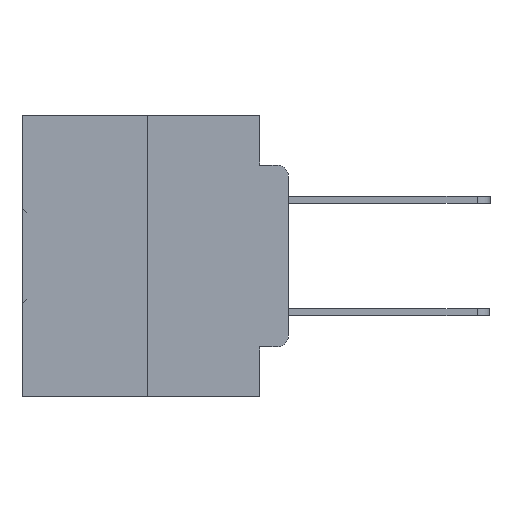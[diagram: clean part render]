
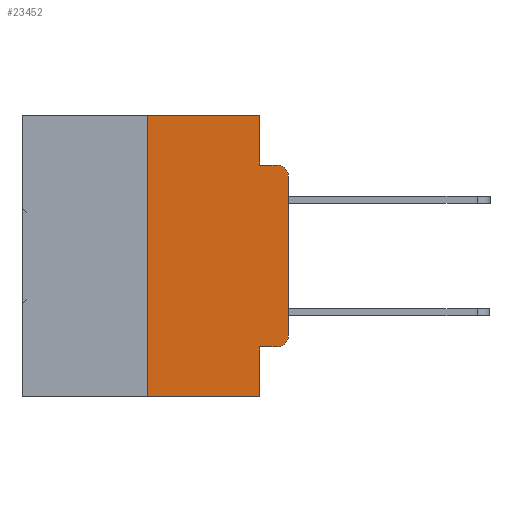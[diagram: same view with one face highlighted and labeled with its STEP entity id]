
A CAD part, left-side view. The second image highlights one B-rep face of the part: STEP entity #23452.
In plain terms, the highlighted planar face has unit normal (-1, 0, 0).
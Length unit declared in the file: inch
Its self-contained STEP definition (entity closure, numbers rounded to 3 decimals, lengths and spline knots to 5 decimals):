
#125 = DIRECTION ( 'NONE',  ( 0., 0., -1. ) ) ;
#289 = VERTEX_POINT ( 'NONE', #16838 ) ;
#683 = LINE ( 'NONE', #22170, #1549 ) ;
#1359 = VERTEX_POINT ( 'NONE', #10719 ) ;
#1549 = VECTOR ( 'NONE', #3094, 39.37008 ) ;
#2025 = EDGE_CURVE ( 'NONE', #9651, #2860, #10734, .T. ) ;
#2363 = DIRECTION ( 'NONE',  ( 0., 0., 1. ) ) ;
#2707 = DIRECTION ( 'NONE',  ( 0., 0., -1. ) ) ;
#2860 = VERTEX_POINT ( 'NONE', #33324 ) ;
#3094 = DIRECTION ( 'NONE',  ( 0., -1., 0. ) ) ;
#3536 = EDGE_CURVE ( 'NONE', #31748, #29244, #20817, .T. ) ;
#4374 = AXIS2_PLACEMENT_3D ( 'NONE', #27597, #30300, #14190 ) ;
#4842 = ORIENTED_EDGE ( 'NONE', *, *, #16041, .T. ) ;
#4948 = CARTESIAN_POINT ( 'NONE',  ( 0., 0.02, -0.1085 ) ) ;
#5234 = LINE ( 'NONE', #31749, #26900 ) ;
#5281 = ORIENTED_EDGE ( 'NONE', *, *, #9708, .F. ) ;
#5683 = EDGE_LOOP ( 'NONE', ( #11292, #4842, #21050, #22722, #11728, #5281, #7027, #21469, #13063, #28225 ) ) ;
#5907 = PLANE ( 'NONE',  #4374 ) ;
#6290 = EDGE_CURVE ( 'NONE', #289, #31748, #683, .T. ) ;
#6337 = VECTOR ( 'NONE', #11534, 39.37008 ) ;
#6367 = VERTEX_POINT ( 'NONE', #27935 ) ;
#6735 = CARTESIAN_POINT ( 'NONE',  ( 0., 0.473, -0.5 ) ) ;
#7027 = ORIENTED_EDGE ( 'NONE', *, *, #26591, .T. ) ;
#7116 = VECTOR ( 'NONE', #9480, 39.37008 ) ;
#7209 = AXIS2_PLACEMENT_3D ( 'NONE', #30746, #14648, #33377 ) ;
#7302 = EDGE_CURVE ( 'NONE', #6367, #24954, #22806, .T. ) ;
#8119 = LINE ( 'NONE', #30561, #21718 ) ;
#8547 = VERTEX_POINT ( 'NONE', #34655 ) ;
#9480 = DIRECTION ( 'NONE',  ( 0., -1., 0. ) ) ;
#9651 = VERTEX_POINT ( 'NONE', #34145 ) ;
#9708 = EDGE_CURVE ( 'NONE', #8547, #289, #5234, .T. ) ;
#9739 = CARTESIAN_POINT ( 'NONE',  ( 0., 0.051, 0. ) ) ;
#9971 = AXIS2_PLACEMENT_3D ( 'NONE', #4948, #16576, #125 ) ;
#10719 = CARTESIAN_POINT ( 'NONE',  ( 0., 0.02, -0.4115 ) ) ;
#10734 = LINE ( 'NONE', #18844, #25955 ) ;
#11292 = ORIENTED_EDGE ( 'NONE', *, *, #2025, .T. ) ;
#11534 = DIRECTION ( 'NONE',  ( 0., 0., -1. ) ) ;
#11652 = EDGE_CURVE ( 'NONE', #1359, #9651, #31369, .T. ) ;
#11728 = ORIENTED_EDGE ( 'NONE', *, *, #6290, .F. ) ;
#12935 = DIRECTION ( 'NONE',  ( 0., 0., 1. ) ) ;
#13063 = ORIENTED_EDGE ( 'NONE', *, *, #29251, .T. ) ;
#14190 = DIRECTION ( 'NONE',  ( 0., 0., -1. ) ) ;
#14440 = CARTESIAN_POINT ( 'NONE',  ( 0., 0.051, 0. ) ) ;
#14648 = DIRECTION ( 'NONE',  ( -1., 0., 0. ) ) ;
#15057 = LINE ( 'NONE', #19139, #29360 ) ;
#16041 = EDGE_CURVE ( 'NONE', #2860, #29183, #16885, .T. ) ;
#16576 = DIRECTION ( 'NONE',  ( -1., 0., 0. ) ) ;
#16838 = CARTESIAN_POINT ( 'NONE',  ( 0., 0.25, 0. ) ) ;
#16885 = CIRCLE ( 'NONE', #9971, 0.02 ) ;
#18844 = CARTESIAN_POINT ( 'NONE',  ( 0., 0., 0. ) ) ;
#18910 = CARTESIAN_POINT ( 'NONE',  ( 0., 0.02, -0.0885 ) ) ;
#19139 = CARTESIAN_POINT ( 'NONE',  ( 0., 0.051, -0.4115 ) ) ;
#20817 = LINE ( 'NONE', #14440, #6337 ) ;
#21050 = ORIENTED_EDGE ( 'NONE', *, *, #21754, .F. ) ;
#21469 = ORIENTED_EDGE ( 'NONE', *, *, #7302, .F. ) ;
#21718 = VECTOR ( 'NONE', #33205, 39.37008 ) ;
#21754 = EDGE_CURVE ( 'NONE', #29244, #29183, #8119, .T. ) ;
#21961 = VECTOR ( 'NONE', #2707, 39.37008 ) ;
#22170 = CARTESIAN_POINT ( 'NONE',  ( 0., 0.473, 0. ) ) ;
#22722 = ORIENTED_EDGE ( 'NONE', *, *, #3536, .F. ) ;
#22806 = LINE ( 'NONE', #32442, #21961 ) ;
#23452 = ADVANCED_FACE ( 'NONE', ( #26668 ), #5907, .F. ) ;
#24312 = DIRECTION ( 'NONE',  ( 0., -1., 0. ) ) ;
#24434 = CARTESIAN_POINT ( 'NONE',  ( 0., 0.051, -0.0885 ) ) ;
#24954 = VERTEX_POINT ( 'NONE', #31985 ) ;
#25955 = VECTOR ( 'NONE', #2363, 39.37008 ) ;
#26591 = EDGE_CURVE ( 'NONE', #8547, #24954, #28718, .T. ) ;
#26668 = FACE_OUTER_BOUND ( 'NONE', #5683, .T. ) ;
#26900 = VECTOR ( 'NONE', #12935, 39.37008 ) ;
#27597 = CARTESIAN_POINT ( 'NONE',  ( 0., 0.473, 0. ) ) ;
#27935 = CARTESIAN_POINT ( 'NONE',  ( 0., 0.051, -0.4115 ) ) ;
#28225 = ORIENTED_EDGE ( 'NONE', *, *, #11652, .T. ) ;
#28718 = LINE ( 'NONE', #6735, #7116 ) ;
#29183 = VERTEX_POINT ( 'NONE', #18910 ) ;
#29244 = VERTEX_POINT ( 'NONE', #24434 ) ;
#29251 = EDGE_CURVE ( 'NONE', #6367, #1359, #15057, .T. ) ;
#29360 = VECTOR ( 'NONE', #24312, 39.37008 ) ;
#30300 = DIRECTION ( 'NONE',  ( 1., 0., 0. ) ) ;
#30561 = CARTESIAN_POINT ( 'NONE',  ( 0., 0.051, -0.0885 ) ) ;
#30746 = CARTESIAN_POINT ( 'NONE',  ( 0., 0.02, -0.3915 ) ) ;
#31369 = CIRCLE ( 'NONE', #7209, 0.02 ) ;
#31748 = VERTEX_POINT ( 'NONE', #9739 ) ;
#31749 = CARTESIAN_POINT ( 'NONE',  ( 0., 0.25, 0. ) ) ;
#31985 = CARTESIAN_POINT ( 'NONE',  ( 0., 0.051, -0.5 ) ) ;
#32442 = CARTESIAN_POINT ( 'NONE',  ( 0., 0.051, 0. ) ) ;
#33205 = DIRECTION ( 'NONE',  ( 0., -1., 0. ) ) ;
#33324 = CARTESIAN_POINT ( 'NONE',  ( 0., 0., -0.1085 ) ) ;
#33377 = DIRECTION ( 'NONE',  ( 0., 0., -1. ) ) ;
#34145 = CARTESIAN_POINT ( 'NONE',  ( 0., 0., -0.3915 ) ) ;
#34655 = CARTESIAN_POINT ( 'NONE',  ( 0., 0.25, -0.5 ) ) ;
